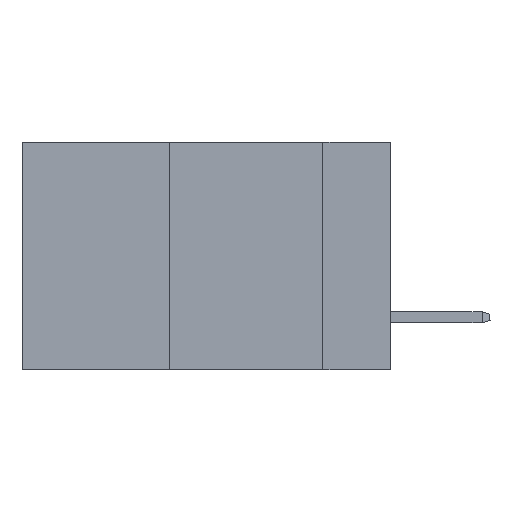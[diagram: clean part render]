
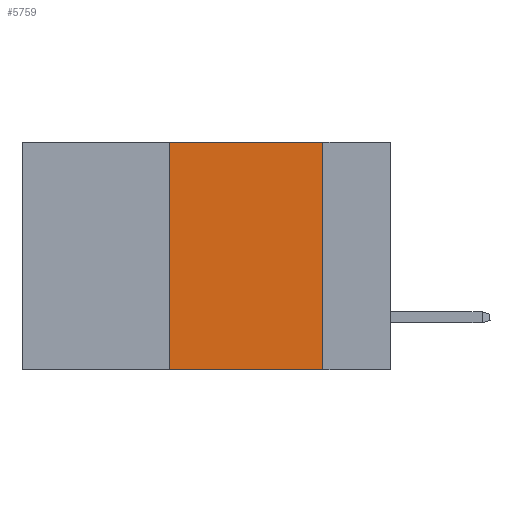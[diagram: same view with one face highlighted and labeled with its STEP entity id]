
A CAD part, left-side view. The second image highlights one B-rep face of the part: STEP entity #5759.
In plain terms, the highlighted planar face has unit normal (-1, 0, 0).
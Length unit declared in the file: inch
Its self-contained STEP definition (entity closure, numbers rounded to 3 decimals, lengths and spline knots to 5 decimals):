
#191 = CARTESIAN_POINT ( 'NONE',  ( 0., 0.11, -0.37 ) ) ;
#219 = EDGE_CURVE ( 'NONE', #5017, #3128, #1555, .T. ) ;
#918 = EDGE_CURVE ( 'NONE', #9433, #5017, #10313, .T. ) ;
#1165 = DIRECTION ( 'NONE',  ( 0., -1., 0. ) ) ;
#1421 = VECTOR ( 'NONE', #1165, 39.37008 ) ;
#1468 = ORIENTED_EDGE ( 'NONE', *, *, #219, .F. ) ;
#1555 = LINE ( 'NONE', #3519, #3908 ) ;
#3128 = VERTEX_POINT ( 'NONE', #191 ) ;
#3403 = DIRECTION ( 'NONE',  ( 0., 0., 1. ) ) ;
#3423 = CARTESIAN_POINT ( 'NONE',  ( 0., 0.6, 0. ) ) ;
#3519 = CARTESIAN_POINT ( 'NONE',  ( 0., 0.11, 0. ) ) ;
#3896 = CARTESIAN_POINT ( 'NONE',  ( 0., 0.6, -0.37 ) ) ;
#3908 = VECTOR ( 'NONE', #8584, 39.37008 ) ;
#4035 = LINE ( 'NONE', #9383, #9157 ) ;
#4092 = CARTESIAN_POINT ( 'NONE',  ( 0., 0.36, -0.37 ) ) ;
#4161 = VECTOR ( 'NONE', #4679, 39.37008 ) ;
#4162 = ORIENTED_EDGE ( 'NONE', *, *, #918, .F. ) ;
#4293 = VERTEX_POINT ( 'NONE', #4092 ) ;
#4679 = DIRECTION ( 'NONE',  ( 0., -1., 0. ) ) ;
#5017 = VERTEX_POINT ( 'NONE', #8667 ) ;
#5199 = AXIS2_PLACEMENT_3D ( 'NONE', #3423, #10118, #7651 ) ;
#5497 = ORIENTED_EDGE ( 'NONE', *, *, #7671, .T. ) ;
#5759 = ADVANCED_FACE ( 'NONE', ( #10516 ), #7618, .F. ) ;
#7084 = CARTESIAN_POINT ( 'NONE',  ( 0., 0.6, 0. ) ) ;
#7618 = PLANE ( 'NONE',  #5199 ) ;
#7651 = DIRECTION ( 'NONE',  ( 0., 0., -1. ) ) ;
#7671 = EDGE_CURVE ( 'NONE', #4293, #3128, #9301, .T. ) ;
#8004 = EDGE_CURVE ( 'NONE', #4293, #9433, #4035, .T. ) ;
#8584 = DIRECTION ( 'NONE',  ( 0., 0., -1. ) ) ;
#8667 = CARTESIAN_POINT ( 'NONE',  ( 0., 0.11, 0. ) ) ;
#9157 = VECTOR ( 'NONE', #3403, 39.37008 ) ;
#9301 = LINE ( 'NONE', #3896, #4161 ) ;
#9383 = CARTESIAN_POINT ( 'NONE',  ( 0., 0.36, 0. ) ) ;
#9433 = VERTEX_POINT ( 'NONE', #10353 ) ;
#9760 = ORIENTED_EDGE ( 'NONE', *, *, #8004, .F. ) ;
#10118 = DIRECTION ( 'NONE',  ( 1., 0., 0. ) ) ;
#10313 = LINE ( 'NONE', #7084, #1421 ) ;
#10353 = CARTESIAN_POINT ( 'NONE',  ( 0., 0.36, 0. ) ) ;
#10516 = FACE_OUTER_BOUND ( 'NONE', #10708, .T. ) ;
#10708 = EDGE_LOOP ( 'NONE', ( #1468, #4162, #9760, #5497 ) ) ;
